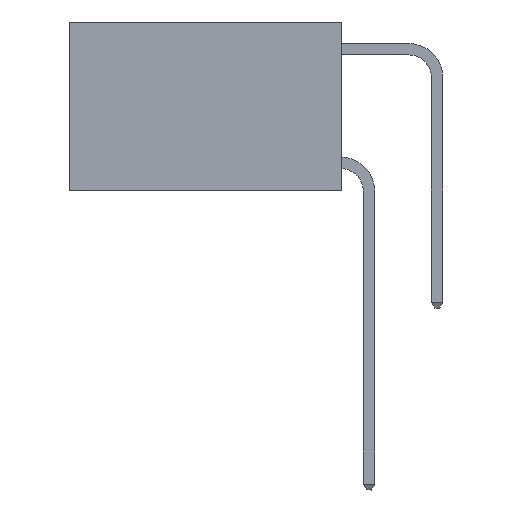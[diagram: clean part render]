
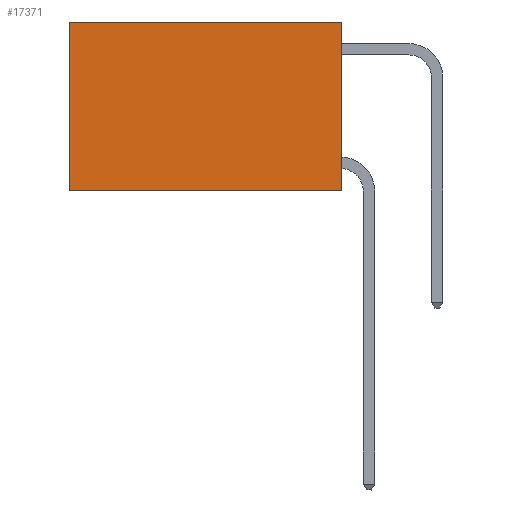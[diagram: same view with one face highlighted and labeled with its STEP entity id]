
A CAD part, left-side view. The second image highlights one B-rep face of the part: STEP entity #17371.
In plain terms, the highlighted planar face has unit normal (-1, 0, 0).
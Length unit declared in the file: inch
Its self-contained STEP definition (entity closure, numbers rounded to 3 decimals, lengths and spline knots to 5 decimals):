
#77 = ORIENTED_EDGE ( 'NONE', *, *, #14085, .F. ) ;
#184 = EDGE_CURVE ( 'NONE', #19015, #14835, #6534, .T. ) ;
#894 = ORIENTED_EDGE ( 'NONE', *, *, #184, .T. ) ;
#1441 = DIRECTION ( 'NONE',  ( 1., 0., 0. ) ) ;
#2143 = VECTOR ( 'NONE', #3968, 39.37008 ) ;
#2780 = LINE ( 'NONE', #4755, #13838 ) ;
#3136 = FACE_OUTER_BOUND ( 'NONE', #7180, .T. ) ;
#3558 = CARTESIAN_POINT ( 'NONE',  ( 0.2625, 0., 0. ) ) ;
#3968 = DIRECTION ( 'NONE',  ( 0., 1., 0. ) ) ;
#4174 = VERTEX_POINT ( 'NONE', #5360 ) ;
#4755 = CARTESIAN_POINT ( 'NONE',  ( 0.2625, 0., 0. ) ) ;
#4985 = ORIENTED_EDGE ( 'NONE', *, *, #8200, .T. ) ;
#5360 = CARTESIAN_POINT ( 'NONE',  ( 0.2625, 0.6, -0.37 ) ) ;
#5410 = CARTESIAN_POINT ( 'NONE',  ( 0.2625, 0.6, 0. ) ) ;
#5831 = VECTOR ( 'NONE', #10630, 39.37008 ) ;
#6089 = CARTESIAN_POINT ( 'NONE',  ( 0.2625, 0., -0.37 ) ) ;
#6281 = LINE ( 'NONE', #15689, #13651 ) ;
#6534 = LINE ( 'NONE', #3558, #2143 ) ;
#7144 = CARTESIAN_POINT ( 'NONE',  ( 0.2625, 0., 0. ) ) ;
#7180 = EDGE_LOOP ( 'NONE', ( #4985, #17604, #77, #894 ) ) ;
#7790 = EDGE_CURVE ( 'NONE', #16200, #4174, #17803, .T. ) ;
#8200 = EDGE_CURVE ( 'NONE', #14835, #4174, #6281, .T. ) ;
#8840 = AXIS2_PLACEMENT_3D ( 'NONE', #7144, #1441, #13168 ) ;
#10088 = PLANE ( 'NONE',  #8840 ) ;
#10630 = DIRECTION ( 'NONE',  ( 0., 1., 0. ) ) ;
#12668 = CARTESIAN_POINT ( 'NONE',  ( 0.2625, 0., -0.37 ) ) ;
#13168 = DIRECTION ( 'NONE',  ( 0., 0., -1. ) ) ;
#13651 = VECTOR ( 'NONE', #17167, 39.37008 ) ;
#13838 = VECTOR ( 'NONE', #17949, 39.37008 ) ;
#14073 = CARTESIAN_POINT ( 'NONE',  ( 0.2625, 0., 0. ) ) ;
#14085 = EDGE_CURVE ( 'NONE', #19015, #16200, #2780, .T. ) ;
#14835 = VERTEX_POINT ( 'NONE', #5410 ) ;
#15689 = CARTESIAN_POINT ( 'NONE',  ( 0.2625, 0.6, 0. ) ) ;
#16200 = VERTEX_POINT ( 'NONE', #12668 ) ;
#17167 = DIRECTION ( 'NONE',  ( 0., 0., -1. ) ) ;
#17371 = ADVANCED_FACE ( 'NONE', ( #3136 ), #10088, .F. ) ;
#17604 = ORIENTED_EDGE ( 'NONE', *, *, #7790, .F. ) ;
#17803 = LINE ( 'NONE', #6089, #5831 ) ;
#17949 = DIRECTION ( 'NONE',  ( 0., 0., -1. ) ) ;
#19015 = VERTEX_POINT ( 'NONE', #14073 ) ;
